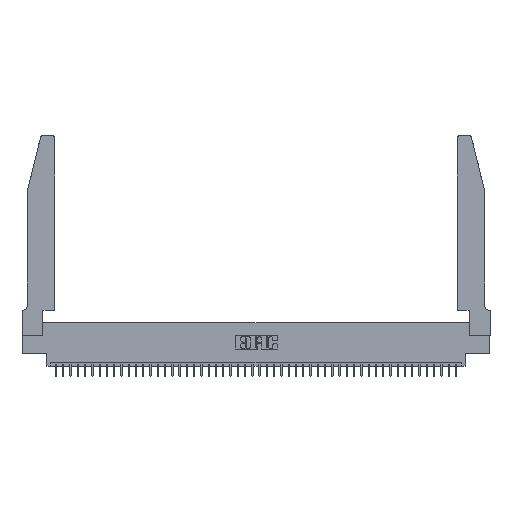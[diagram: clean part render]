
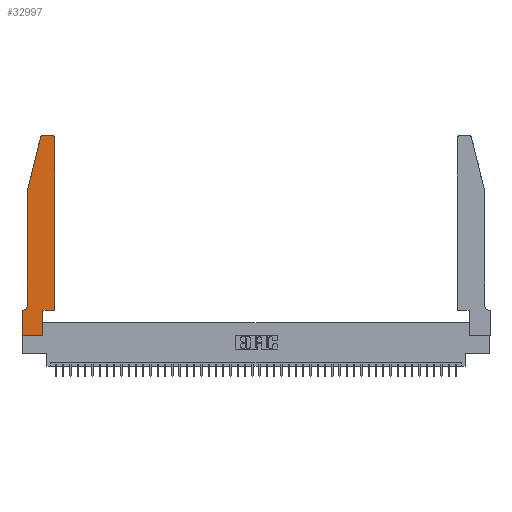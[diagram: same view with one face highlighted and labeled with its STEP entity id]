
A CAD part, top view. The second image highlights one B-rep face of the part: STEP entity #32997.
In plain terms, the highlighted planar face has unit normal (0, 0, 1).
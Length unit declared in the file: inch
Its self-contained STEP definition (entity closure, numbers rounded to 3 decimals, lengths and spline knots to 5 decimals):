
#300 = CARTESIAN_POINT ( 'NONE',  ( 0., 0., 0.37 ) ) ;
#954 = LINE ( 'NONE', #23381, #41165 ) ;
#965 = VERTEX_POINT ( 'NONE', #46381 ) ;
#1362 = VECTOR ( 'NONE', #33546, 39.37008 ) ;
#1495 = CIRCLE ( 'NONE', #46330, 0.03 ) ;
#1603 = VERTEX_POINT ( 'NONE', #15332 ) ;
#1938 = ORIENTED_EDGE ( 'NONE', *, *, #33729, .T. ) ;
#2263 = CARTESIAN_POINT ( 'NONE',  ( 0.0055, 0.42, 0.37 ) ) ;
#3000 = CARTESIAN_POINT ( 'NONE',  ( 0., 0.35, 0.37 ) ) ;
#3217 = VERTEX_POINT ( 'NONE', #10411 ) ;
#3483 = EDGE_CURVE ( 'NONE', #19047, #3217, #46824, .T. ) ;
#4425 = CARTESIAN_POINT ( 'NONE',  ( 0.0755, 2., 0.37 ) ) ;
#4730 = LINE ( 'NONE', #33776, #15033 ) ;
#4809 = VECTOR ( 'NONE', #24855, 39.37008 ) ;
#4953 = DIRECTION ( 'NONE',  ( 0., -1., 0. ) ) ;
#5199 = VECTOR ( 'NONE', #24061, 39.37008 ) ;
#5505 = DIRECTION ( 'NONE',  ( -1., 0., 0. ) ) ;
#5575 = VERTEX_POINT ( 'NONE', #9865 ) ;
#5924 = ORIENTED_EDGE ( 'NONE', *, *, #3483, .T. ) ;
#6773 = LINE ( 'NONE', #14377, #4809 ) ;
#8067 = EDGE_CURVE ( 'NONE', #26523, #44955, #1495, .T. ) ;
#8871 = CARTESIAN_POINT ( 'NONE',  ( 0.0755, 0.42, 0.37 ) ) ;
#9699 = VECTOR ( 'NONE', #28492, 39.37008 ) ;
#9865 = CARTESIAN_POINT ( 'NONE',  ( 0.4205, 2.75, 0.37 ) ) ;
#10188 = CARTESIAN_POINT ( 'NONE',  ( 0., 0.35, 0.37 ) ) ;
#10411 = CARTESIAN_POINT ( 'NONE',  ( 0.4505, 0.35, 0.37 ) ) ;
#10872 = VECTOR ( 'NONE', #39633, 39.37008 ) ;
#11894 = EDGE_CURVE ( 'NONE', #5575, #26523, #6773, .T. ) ;
#11955 = CARTESIAN_POINT ( 'NONE',  ( 0.4505, 2.72, 0.37 ) ) ;
#12818 = AXIS2_PLACEMENT_3D ( 'NONE', #32474, #42973, #32712 ) ;
#13087 = VERTEX_POINT ( 'NONE', #3000 ) ;
#13269 = LINE ( 'NONE', #20428, #9699 ) ;
#13984 = DIRECTION ( 'NONE',  ( 1., 0., 0. ) ) ;
#14214 = EDGE_CURVE ( 'NONE', #13087, #39188, #4730, .T. ) ;
#14377 = CARTESIAN_POINT ( 'NONE',  ( 0.2605, 2.75, 0.37 ) ) ;
#14460 = EDGE_CURVE ( 'NONE', #3217, #19314, #13269, .T. ) ;
#14483 = CARTESIAN_POINT ( 'NONE',  ( 0.4505, 0.35, 0.37 ) ) ;
#15033 = VECTOR ( 'NONE', #4953, 39.37008 ) ;
#15332 = CARTESIAN_POINT ( 'NONE',  ( 0.2865, 0., 0.37 ) ) ;
#15718 = ORIENTED_EDGE ( 'NONE', *, *, #34790, .T. ) ;
#17169 = CARTESIAN_POINT ( 'NONE',  ( 0.0755, 2., 0.37 ) ) ;
#17254 = CARTESIAN_POINT ( 'NONE',  ( 0.25487, 2.72718, 0.37 ) ) ;
#17526 = VECTOR ( 'NONE', #29911, 39.37008 ) ;
#18031 = FACE_OUTER_BOUND ( 'NONE', #45196, .T. ) ;
#18282 = ORIENTED_EDGE ( 'NONE', *, *, #14214, .T. ) ;
#18637 = CARTESIAN_POINT ( 'NONE',  ( 0.284, 2.72, 0.37 ) ) ;
#19047 = VERTEX_POINT ( 'NONE', #35551 ) ;
#19065 = ORIENTED_EDGE ( 'NONE', *, *, #8067, .T. ) ;
#19281 = LINE ( 'NONE', #33780, #1362 ) ;
#19314 = VERTEX_POINT ( 'NONE', #11955 ) ;
#20078 = EDGE_CURVE ( 'NONE', #39582, #36172, #44423, .T. ) ;
#20090 = ORIENTED_EDGE ( 'NONE', *, *, #14460, .T. ) ;
#20428 = CARTESIAN_POINT ( 'NONE',  ( 0.4505, 0.35, 0.37 ) ) ;
#22696 = DIRECTION ( 'NONE',  ( 0., 0., 1. ) ) ;
#23381 = CARTESIAN_POINT ( 'NONE',  ( 0.0755, 0.35, 0.37 ) ) ;
#24059 = VECTOR ( 'NONE', #35667, 39.37008 ) ;
#24061 = DIRECTION ( 'NONE',  ( -0.239, -0.971, 0. ) ) ;
#24182 = DIRECTION ( 'NONE',  ( -1., 0., 0. ) ) ;
#24855 = DIRECTION ( 'NONE',  ( -1., 0., 0. ) ) ;
#25081 = ORIENTED_EDGE ( 'NONE', *, *, #39793, .T. ) ;
#25146 = LINE ( 'NONE', #43231, #10872 ) ;
#26523 = VERTEX_POINT ( 'NONE', #38452 ) ;
#27403 = ORIENTED_EDGE ( 'NONE', *, *, #33996, .T. ) ;
#28489 = PLANE ( 'NONE',  #42495 ) ;
#28492 = DIRECTION ( 'NONE',  ( 0., 1., 0. ) ) ;
#29911 = DIRECTION ( 'NONE',  ( 0., -1., 0. ) ) ;
#31833 = CIRCLE ( 'NONE', #12818, 0.03 ) ;
#32474 = CARTESIAN_POINT ( 'NONE',  ( 0.4205, 2.72, 0.37 ) ) ;
#32682 = ORIENTED_EDGE ( 'NONE', *, *, #34619, .T. ) ;
#32712 = DIRECTION ( 'NONE',  ( 1., 0., 0. ) ) ;
#32997 = ADVANCED_FACE ( 'NONE', ( #18031 ), #28489, .T. ) ;
#33150 = DIRECTION ( 'NONE',  ( 1., 0., 0. ) ) ;
#33546 = DIRECTION ( 'NONE',  ( 1., 0., 0. ) ) ;
#33729 = EDGE_CURVE ( 'NONE', #44955, #39582, #35238, .T. ) ;
#33776 = CARTESIAN_POINT ( 'NONE',  ( 0., 0., 0.37 ) ) ;
#33780 = CARTESIAN_POINT ( 'NONE',  ( 0., 0., 0.37 ) ) ;
#33996 = EDGE_CURVE ( 'NONE', #39188, #1603, #19281, .T. ) ;
#34619 = EDGE_CURVE ( 'NONE', #36172, #965, #35623, .T. ) ;
#34790 = EDGE_CURVE ( 'NONE', #19314, #5575, #31833, .T. ) ;
#34913 = ORIENTED_EDGE ( 'NONE', *, *, #37769, .T. ) ;
#35238 = LINE ( 'NONE', #17169, #5199 ) ;
#35551 = CARTESIAN_POINT ( 'NONE',  ( 0.2865, 0.35, 0.37 ) ) ;
#35623 = CIRCLE ( 'NONE', #37911, 0.07 ) ;
#35667 = DIRECTION ( 'NONE',  ( 1., 0., 0. ) ) ;
#36172 = VERTEX_POINT ( 'NONE', #8871 ) ;
#37769 = EDGE_CURVE ( 'NONE', #965, #13087, #954, .T. ) ;
#37911 = AXIS2_PLACEMENT_3D ( 'NONE', #2263, #38916, #24182 ) ;
#38452 = CARTESIAN_POINT ( 'NONE',  ( 0.284, 2.75, 0.37 ) ) ;
#38916 = DIRECTION ( 'NONE',  ( 0., 0., -1. ) ) ;
#39188 = VERTEX_POINT ( 'NONE', #300 ) ;
#39496 = ORIENTED_EDGE ( 'NONE', *, *, #20078, .T. ) ;
#39582 = VERTEX_POINT ( 'NONE', #45150 ) ;
#39633 = DIRECTION ( 'NONE',  ( 0., 1., 0. ) ) ;
#39793 = EDGE_CURVE ( 'NONE', #1603, #19047, #25146, .T. ) ;
#41165 = VECTOR ( 'NONE', #5505, 39.37008 ) ;
#42495 = AXIS2_PLACEMENT_3D ( 'NONE', #10188, #46801, #13984 ) ;
#42973 = DIRECTION ( 'NONE',  ( 0., 0., 1. ) ) ;
#43231 = CARTESIAN_POINT ( 'NONE',  ( 0.2865, 0.35, 0.37 ) ) ;
#44423 = LINE ( 'NONE', #4425, #17526 ) ;
#44955 = VERTEX_POINT ( 'NONE', #17254 ) ;
#45150 = CARTESIAN_POINT ( 'NONE',  ( 0.0755, 2., 0.37 ) ) ;
#45196 = EDGE_LOOP ( 'NONE', ( #45664, #19065, #1938, #39496, #32682, #34913, #18282, #27403, #25081, #5924, #20090, #15718 ) ) ;
#45664 = ORIENTED_EDGE ( 'NONE', *, *, #11894, .T. ) ;
#46330 = AXIS2_PLACEMENT_3D ( 'NONE', #18637, #22696, #33150 ) ;
#46381 = CARTESIAN_POINT ( 'NONE',  ( 0.0055, 0.35, 0.37 ) ) ;
#46801 = DIRECTION ( 'NONE',  ( 0., 0., 1. ) ) ;
#46824 = LINE ( 'NONE', #14483, #24059 ) ;
